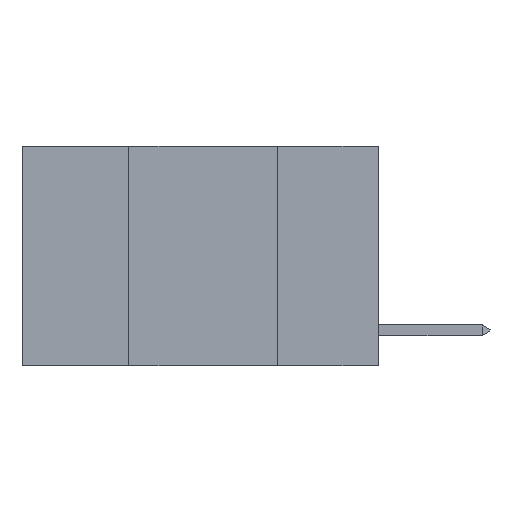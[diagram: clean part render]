
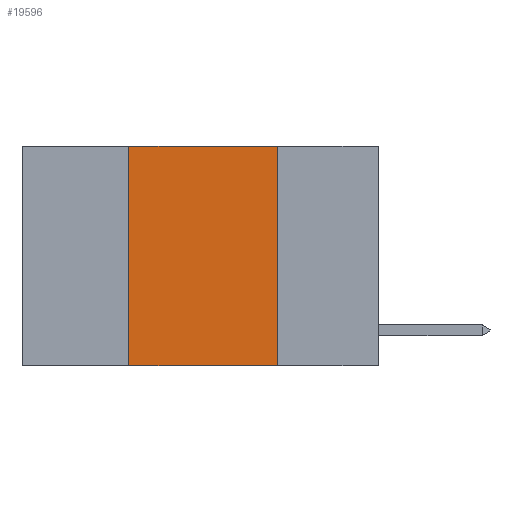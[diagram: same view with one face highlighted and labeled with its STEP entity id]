
A CAD part, left-side view. The second image highlights one B-rep face of the part: STEP entity #19596.
In plain terms, the highlighted planar face has unit normal (-1, 0, 0).
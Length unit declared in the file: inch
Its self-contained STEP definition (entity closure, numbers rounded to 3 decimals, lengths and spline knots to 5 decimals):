
#238 = LINE ( 'NONE', #15302, #12914 ) ;
#379 = DIRECTION ( 'NONE',  ( 0., 0., -1. ) ) ;
#387 = VECTOR ( 'NONE', #21936, 39.37008 ) ;
#1088 = ORIENTED_EDGE ( 'NONE', *, *, #24324, .F. ) ;
#2564 = VERTEX_POINT ( 'NONE', #7933 ) ;
#3537 = DIRECTION ( 'NONE',  ( 0., -1., 0. ) ) ;
#4055 = PLANE ( 'NONE',  #4436 ) ;
#4436 = AXIS2_PLACEMENT_3D ( 'NONE', #19108, #9710, #379 ) ;
#4493 = CARTESIAN_POINT ( 'NONE',  ( 0., 0.6, -0.37 ) ) ;
#4717 = CARTESIAN_POINT ( 'NONE',  ( 0., 0.6, 0. ) ) ;
#5907 = DIRECTION ( 'NONE',  ( 0., 0., -1. ) ) ;
#6746 = ORIENTED_EDGE ( 'NONE', *, *, #21851, .F. ) ;
#7933 = CARTESIAN_POINT ( 'NONE',  ( 0., 0.42, 0. ) ) ;
#8765 = LINE ( 'NONE', #14445, #387 ) ;
#9634 = VECTOR ( 'NONE', #17383, 39.37008 ) ;
#9710 = DIRECTION ( 'NONE',  ( 1., 0., 0. ) ) ;
#10880 = LINE ( 'NONE', #4717, #19035 ) ;
#12057 = VERTEX_POINT ( 'NONE', #21977 ) ;
#12655 = EDGE_LOOP ( 'NONE', ( #1088, #22596, #6746, #23282 ) ) ;
#12914 = VECTOR ( 'NONE', #5907, 39.37008 ) ;
#13885 = LINE ( 'NONE', #4493, #9634 ) ;
#14445 = CARTESIAN_POINT ( 'NONE',  ( 0., 0.42, 0. ) ) ;
#15302 = CARTESIAN_POINT ( 'NONE',  ( 0., 0.17, 0. ) ) ;
#17383 = DIRECTION ( 'NONE',  ( 0., -1., 0. ) ) ;
#17533 = EDGE_CURVE ( 'NONE', #12057, #20050, #13885, .T. ) ;
#19035 = VECTOR ( 'NONE', #3537, 39.37008 ) ;
#19108 = CARTESIAN_POINT ( 'NONE',  ( 0., 0.6, 0. ) ) ;
#19445 = CARTESIAN_POINT ( 'NONE',  ( 0., 0.17, -0.37 ) ) ;
#19596 = ADVANCED_FACE ( 'NONE', ( #20932 ), #4055, .F. ) ;
#19756 = EDGE_CURVE ( 'NONE', #2564, #20377, #10880, .T. ) ;
#20050 = VERTEX_POINT ( 'NONE', #19445 ) ;
#20377 = VERTEX_POINT ( 'NONE', #23410 ) ;
#20932 = FACE_OUTER_BOUND ( 'NONE', #12655, .T. ) ;
#21851 = EDGE_CURVE ( 'NONE', #12057, #2564, #8765, .T. ) ;
#21936 = DIRECTION ( 'NONE',  ( 0., 0., 1. ) ) ;
#21977 = CARTESIAN_POINT ( 'NONE',  ( 0., 0.42, -0.37 ) ) ;
#22596 = ORIENTED_EDGE ( 'NONE', *, *, #19756, .F. ) ;
#23282 = ORIENTED_EDGE ( 'NONE', *, *, #17533, .T. ) ;
#23410 = CARTESIAN_POINT ( 'NONE',  ( 0., 0.17, 0. ) ) ;
#24324 = EDGE_CURVE ( 'NONE', #20377, #20050, #238, .T. ) ;
